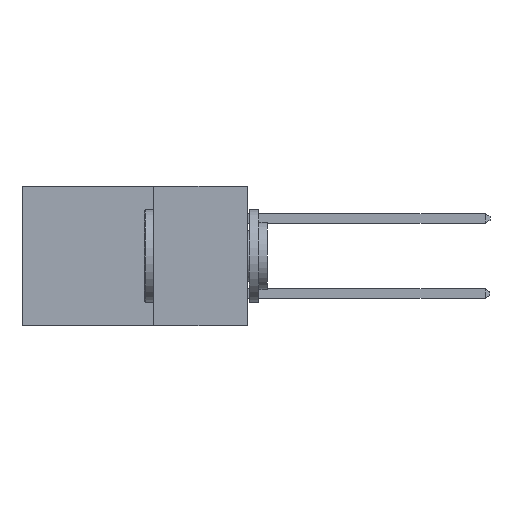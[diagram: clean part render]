
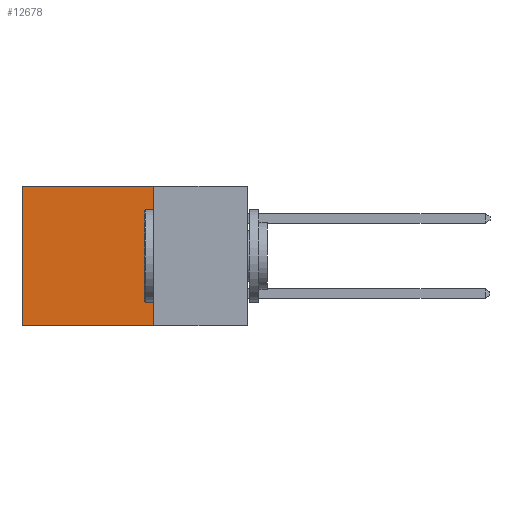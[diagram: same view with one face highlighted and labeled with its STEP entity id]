
A CAD part, left-side view. The second image highlights one B-rep face of the part: STEP entity #12678.
In plain terms, the highlighted planar face has unit normal (-1, 0, 0).
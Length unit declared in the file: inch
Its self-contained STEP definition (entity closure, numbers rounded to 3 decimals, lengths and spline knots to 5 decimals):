
#270 = PLANE ( 'NONE',  #21984 ) ;
#284 = LINE ( 'NONE', #22327, #13851 ) ;
#1425 = ORIENTED_EDGE ( 'NONE', *, *, #18651, .F. ) ;
#1533 = CARTESIAN_POINT ( 'NONE',  ( 0.298, 0.25, -0.37 ) ) ;
#1623 = CARTESIAN_POINT ( 'NONE',  ( 0.298, 0.6, -0.37 ) ) ;
#1898 = LINE ( 'NONE', #1533, #10758 ) ;
#1958 = ORIENTED_EDGE ( 'NONE', *, *, #17681, .T. ) ;
#2063 = DIRECTION ( 'NONE',  ( 1., 0., 0. ) ) ;
#2416 = FACE_OUTER_BOUND ( 'NONE', #19388, .T. ) ;
#2972 = DIRECTION ( 'NONE',  ( 0., 0., -1. ) ) ;
#4059 = CARTESIAN_POINT ( 'NONE',  ( 0.298, 0.25, 0. ) ) ;
#4197 = VERTEX_POINT ( 'NONE', #21011 ) ;
#4731 = VECTOR ( 'NONE', #11082, 39.37008 ) ;
#5539 = CARTESIAN_POINT ( 'NONE',  ( 0.298, 0.25, 0. ) ) ;
#6649 = VECTOR ( 'NONE', #9935, 39.37008 ) ;
#6874 = DIRECTION ( 'NONE',  ( 0., 1., 0. ) ) ;
#9332 = CARTESIAN_POINT ( 'NONE',  ( 0.298, 0.6, 0. ) ) ;
#9935 = DIRECTION ( 'NONE',  ( 0., 0., -1. ) ) ;
#10758 = VECTOR ( 'NONE', #6874, 39.37008 ) ;
#10899 = EDGE_CURVE ( 'NONE', #19782, #13994, #11351, .T. ) ;
#11082 = DIRECTION ( 'NONE',  ( 0., 1., 0. ) ) ;
#11351 = LINE ( 'NONE', #18674, #6649 ) ;
#11736 = ORIENTED_EDGE ( 'NONE', *, *, #22129, .F. ) ;
#12678 = ADVANCED_FACE ( 'NONE', ( #2416 ), #270, .F. ) ;
#13851 = VECTOR ( 'NONE', #2972, 39.37008 ) ;
#13994 = VERTEX_POINT ( 'NONE', #1623 ) ;
#14431 = DIRECTION ( 'NONE',  ( 0., 0., -1. ) ) ;
#17681 = EDGE_CURVE ( 'NONE', #4197, #19782, #22448, .T. ) ;
#18554 = VERTEX_POINT ( 'NONE', #22511 ) ;
#18651 = EDGE_CURVE ( 'NONE', #18554, #13994, #1898, .T. ) ;
#18674 = CARTESIAN_POINT ( 'NONE',  ( 0.298, 0.6, 0. ) ) ;
#19388 = EDGE_LOOP ( 'NONE', ( #21499, #1425, #11736, #1958 ) ) ;
#19782 = VERTEX_POINT ( 'NONE', #9332 ) ;
#21011 = CARTESIAN_POINT ( 'NONE',  ( 0.298, 0.25, 0. ) ) ;
#21499 = ORIENTED_EDGE ( 'NONE', *, *, #10899, .T. ) ;
#21984 = AXIS2_PLACEMENT_3D ( 'NONE', #5539, #2063, #14431 ) ;
#22129 = EDGE_CURVE ( 'NONE', #4197, #18554, #284, .T. ) ;
#22327 = CARTESIAN_POINT ( 'NONE',  ( 0.298, 0.25, 0. ) ) ;
#22448 = LINE ( 'NONE', #4059, #4731 ) ;
#22511 = CARTESIAN_POINT ( 'NONE',  ( 0.298, 0.25, -0.37 ) ) ;
